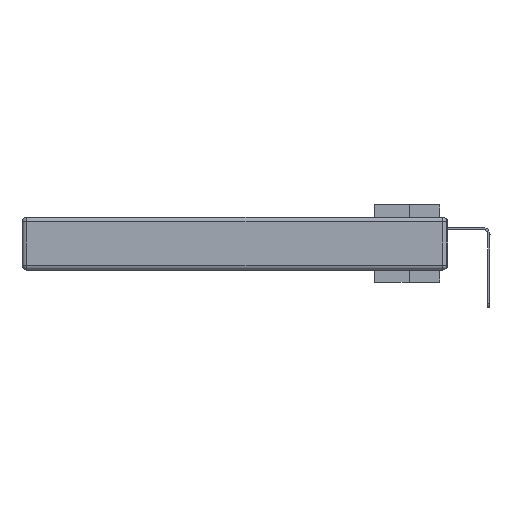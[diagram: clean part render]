
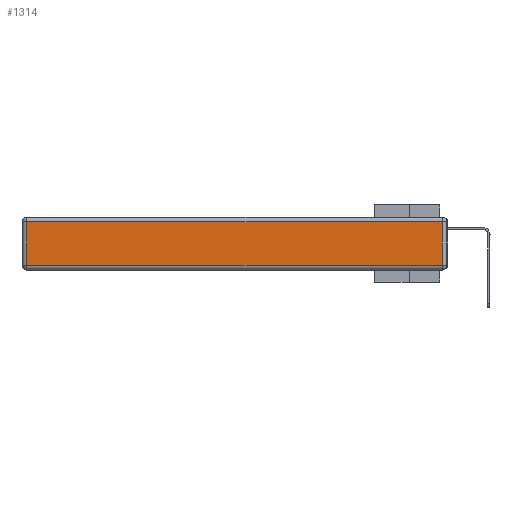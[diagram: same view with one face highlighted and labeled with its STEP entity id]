
A CAD part, left-side view. The second image highlights one B-rep face of the part: STEP entity #1314.
In plain terms, the highlighted planar face has unit normal (-1, 0, 0).
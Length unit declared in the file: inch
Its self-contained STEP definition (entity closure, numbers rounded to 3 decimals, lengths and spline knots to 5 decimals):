
#379 = ORIENTED_EDGE ( 'NONE', *, *, #29274, .T. ) ;
#763 = DIRECTION ( 'NONE',  ( 0., 0., -1. ) ) ;
#1093 = LINE ( 'NONE', #28787, #19375 ) ;
#1289 = VERTEX_POINT ( 'NONE', #26637 ) ;
#1314 = ADVANCED_FACE ( 'NONE', ( #30228 ), #19434, .T. ) ;
#4080 = EDGE_LOOP ( 'NONE', ( #12300, #27532, #7959, #379 ) ) ;
#4897 = EDGE_CURVE ( 'NONE', #23828, #24060, #1093, .T. ) ;
#5635 = CARTESIAN_POINT ( 'NONE',  ( 0., 2.72, -0.03 ) ) ;
#6231 = AXIS2_PLACEMENT_3D ( 'NONE', #21232, #21632, #30980 ) ;
#6701 = VECTOR ( 'NONE', #18831, 39.37008 ) ;
#7959 = ORIENTED_EDGE ( 'NONE', *, *, #4897, .T. ) ;
#8801 = CARTESIAN_POINT ( 'NONE',  ( 0., 0.03, -0.343 ) ) ;
#9465 = VERTEX_POINT ( 'NONE', #29963 ) ;
#12300 = ORIENTED_EDGE ( 'NONE', *, *, #13649, .T. ) ;
#12598 = EDGE_CURVE ( 'NONE', #1289, #23828, #17413, .T. ) ;
#13649 = EDGE_CURVE ( 'NONE', #9465, #1289, #21887, .T. ) ;
#14975 = VECTOR ( 'NONE', #22615, 39.37008 ) ;
#17306 = LINE ( 'NONE', #18048, #31040 ) ;
#17413 = LINE ( 'NONE', #8801, #6701 ) ;
#18048 = CARTESIAN_POINT ( 'NONE',  ( 0., 2.72, -0.343 ) ) ;
#18831 = DIRECTION ( 'NONE',  ( 0., 0., 1. ) ) ;
#19007 = CARTESIAN_POINT ( 'NONE',  ( 0., 0.03, -0.03 ) ) ;
#19375 = VECTOR ( 'NONE', #29200, 39.37008 ) ;
#19434 = PLANE ( 'NONE',  #6231 ) ;
#21232 = CARTESIAN_POINT ( 'NONE',  ( 0., 0., -0.343 ) ) ;
#21632 = DIRECTION ( 'NONE',  ( -1., 0., 0. ) ) ;
#21887 = LINE ( 'NONE', #27693, #14975 ) ;
#22615 = DIRECTION ( 'NONE',  ( 0., -1., 0. ) ) ;
#23828 = VERTEX_POINT ( 'NONE', #19007 ) ;
#24060 = VERTEX_POINT ( 'NONE', #5635 ) ;
#26637 = CARTESIAN_POINT ( 'NONE',  ( 0., 0.03, -0.313 ) ) ;
#27532 = ORIENTED_EDGE ( 'NONE', *, *, #12598, .T. ) ;
#27693 = CARTESIAN_POINT ( 'NONE',  ( 0., 0., -0.313 ) ) ;
#28787 = CARTESIAN_POINT ( 'NONE',  ( 0., 2.75, -0.03 ) ) ;
#29200 = DIRECTION ( 'NONE',  ( 0., 1., 0. ) ) ;
#29274 = EDGE_CURVE ( 'NONE', #24060, #9465, #17306, .T. ) ;
#29963 = CARTESIAN_POINT ( 'NONE',  ( 0., 2.72, -0.313 ) ) ;
#30228 = FACE_OUTER_BOUND ( 'NONE', #4080, .T. ) ;
#30980 = DIRECTION ( 'NONE',  ( 0., 0., 1. ) ) ;
#31040 = VECTOR ( 'NONE', #763, 39.37008 ) ;
